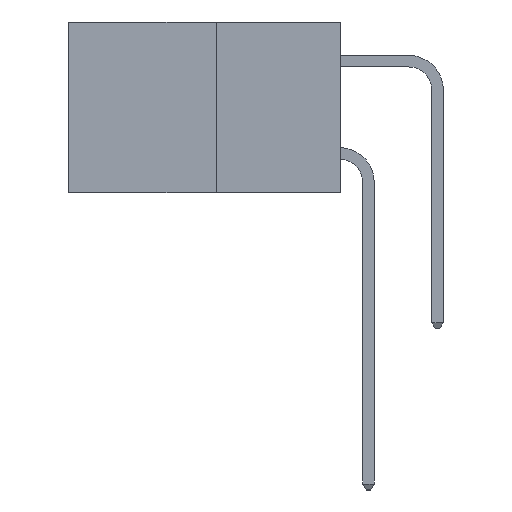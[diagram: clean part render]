
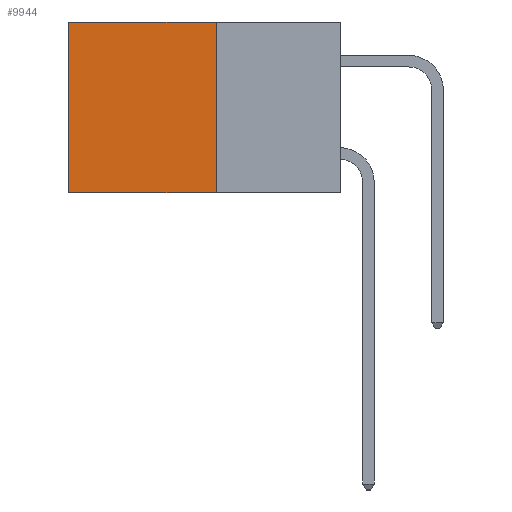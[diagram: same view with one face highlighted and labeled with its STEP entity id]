
A CAD part, left-side view. The second image highlights one B-rep face of the part: STEP entity #9944.
In plain terms, the highlighted planar face has unit normal (-1, 0, 0).
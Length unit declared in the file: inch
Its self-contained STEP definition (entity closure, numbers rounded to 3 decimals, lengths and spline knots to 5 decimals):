
#151 = EDGE_CURVE ( 'NONE', #16055, #1818, #14503, .T. ) ;
#1091 = LINE ( 'NONE', #7845, #15067 ) ;
#1818 = VERTEX_POINT ( 'NONE', #10096 ) ;
#1868 = VERTEX_POINT ( 'NONE', #6128 ) ;
#1898 = EDGE_LOOP ( 'NONE', ( #6301, #7477, #9664, #9838 ) ) ;
#2385 = AXIS2_PLACEMENT_3D ( 'NONE', #14975, #8063, #17607 ) ;
#2677 = CARTESIAN_POINT ( 'NONE',  ( 0.277, 0.59, -0.37 ) ) ;
#3233 = VECTOR ( 'NONE', #12521, 39.37008 ) ;
#3893 = CARTESIAN_POINT ( 'NONE',  ( 0.277, 0.27, -0.37 ) ) ;
#3994 = EDGE_CURVE ( 'NONE', #1868, #17144, #1091, .T. ) ;
#4041 = CARTESIAN_POINT ( 'NONE',  ( 0.277, 0.27, -0.37 ) ) ;
#5343 = DIRECTION ( 'NONE',  ( 0., 0., -1. ) ) ;
#6128 = CARTESIAN_POINT ( 'NONE',  ( 0.277, 0.27, 0. ) ) ;
#6301 = ORIENTED_EDGE ( 'NONE', *, *, #17223, .T. ) ;
#6656 = PLANE ( 'NONE',  #2385 ) ;
#7477 = ORIENTED_EDGE ( 'NONE', *, *, #151, .F. ) ;
#7538 = VECTOR ( 'NONE', #9112, 39.37008 ) ;
#7845 = CARTESIAN_POINT ( 'NONE',  ( 0.277, 0.27, 0. ) ) ;
#8063 = DIRECTION ( 'NONE',  ( 1., 0., 0. ) ) ;
#8077 = CARTESIAN_POINT ( 'NONE',  ( 0.277, 0.59, 0. ) ) ;
#9112 = DIRECTION ( 'NONE',  ( 0., 1., 0. ) ) ;
#9664 = ORIENTED_EDGE ( 'NONE', *, *, #16575, .F. ) ;
#9838 = ORIENTED_EDGE ( 'NONE', *, *, #3994, .T. ) ;
#9944 = ADVANCED_FACE ( 'NONE', ( #11907 ), #6656, .F. ) ;
#10096 = CARTESIAN_POINT ( 'NONE',  ( 0.277, 0.59, -0.37 ) ) ;
#11183 = LINE ( 'NONE', #3893, #16114 ) ;
#11907 = FACE_OUTER_BOUND ( 'NONE', #1898, .T. ) ;
#12521 = DIRECTION ( 'NONE',  ( 0., 0., -1. ) ) ;
#13483 = CARTESIAN_POINT ( 'NONE',  ( 0.277, 0.27, -0.37 ) ) ;
#14503 = LINE ( 'NONE', #13483, #7538 ) ;
#14975 = CARTESIAN_POINT ( 'NONE',  ( 0.277, 0.27, -0.37 ) ) ;
#15067 = VECTOR ( 'NONE', #17139, 39.37008 ) ;
#16055 = VERTEX_POINT ( 'NONE', #4041 ) ;
#16114 = VECTOR ( 'NONE', #5343, 39.37008 ) ;
#16575 = EDGE_CURVE ( 'NONE', #1868, #16055, #11183, .T. ) ;
#17139 = DIRECTION ( 'NONE',  ( 0., 1., 0. ) ) ;
#17144 = VERTEX_POINT ( 'NONE', #8077 ) ;
#17223 = EDGE_CURVE ( 'NONE', #17144, #1818, #17455, .T. ) ;
#17455 = LINE ( 'NONE', #2677, #3233 ) ;
#17607 = DIRECTION ( 'NONE',  ( 0., 0., -1. ) ) ;
